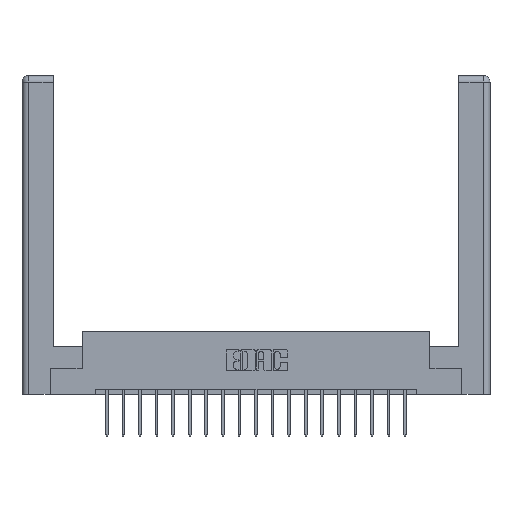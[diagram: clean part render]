
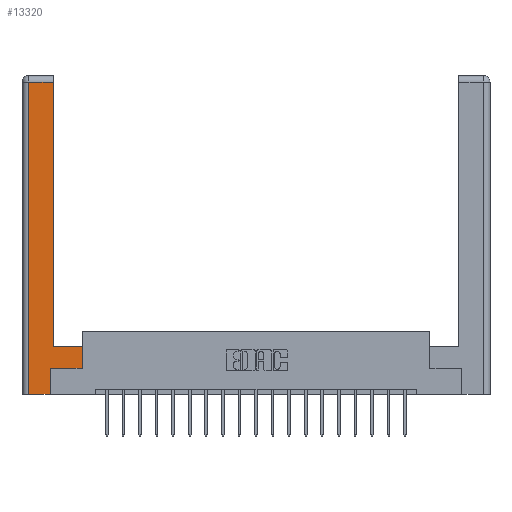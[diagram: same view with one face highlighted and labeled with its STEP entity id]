
A CAD part, top view. The second image highlights one B-rep face of the part: STEP entity #13320.
In plain terms, the highlighted planar face has unit normal (0, 0, 1).
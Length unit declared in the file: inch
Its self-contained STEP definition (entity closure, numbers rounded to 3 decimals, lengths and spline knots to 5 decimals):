
#683 = CARTESIAN_POINT ( 'NONE',  ( 0.295, 0.45, 0. ) ) ;
#913 = VECTOR ( 'NONE', #14217, 39.37008 ) ;
#1145 = CARTESIAN_POINT ( 'NONE',  ( 0.565, 0.245, 0. ) ) ;
#1337 = VERTEX_POINT ( 'NONE', #8075 ) ;
#1497 = DIRECTION ( 'NONE',  ( 0., -1., 0. ) ) ;
#1856 = CARTESIAN_POINT ( 'NONE',  ( 0.295, 2.94, 0. ) ) ;
#2027 = CARTESIAN_POINT ( 'NONE',  ( 0.565, 0.45, 0. ) ) ;
#2874 = EDGE_CURVE ( 'NONE', #4989, #14697, #19048, .T. ) ;
#3342 = ORIENTED_EDGE ( 'NONE', *, *, #14448, .T. ) ;
#3668 = DIRECTION ( 'NONE',  ( -1., 0., 0. ) ) ;
#3799 = PLANE ( 'NONE',  #14968 ) ;
#3950 = EDGE_CURVE ( 'NONE', #11197, #4989, #19739, .T. ) ;
#4392 = LINE ( 'NONE', #13558, #9795 ) ;
#4989 = VERTEX_POINT ( 'NONE', #2027 ) ;
#5073 = VECTOR ( 'NONE', #1497, 39.37008 ) ;
#5989 = EDGE_CURVE ( 'NONE', #13830, #11197, #15475, .T. ) ;
#6300 = ORIENTED_EDGE ( 'NONE', *, *, #15466, .T. ) ;
#6394 = VECTOR ( 'NONE', #11807, 39.37008 ) ;
#7390 = VERTEX_POINT ( 'NONE', #1856 ) ;
#7512 = EDGE_CURVE ( 'NONE', #1337, #7994, #4392, .T. ) ;
#7767 = CARTESIAN_POINT ( 'NONE',  ( 0.565, 0.45, 0. ) ) ;
#7864 = CARTESIAN_POINT ( 'NONE',  ( 0.0615, 2.94, 0. ) ) ;
#7979 = VECTOR ( 'NONE', #8437, 39.37008 ) ;
#7994 = VERTEX_POINT ( 'NONE', #13193 ) ;
#8042 = CARTESIAN_POINT ( 'NONE',  ( 0.265, 0.245, 0. ) ) ;
#8075 = CARTESIAN_POINT ( 'NONE',  ( 0.0615, 0., 0. ) ) ;
#8390 = CARTESIAN_POINT ( 'NONE',  ( 0., 0., 0. ) ) ;
#8437 = DIRECTION ( 'NONE',  ( 0., 1., 0. ) ) ;
#9795 = VECTOR ( 'NONE', #15606, 39.37008 ) ;
#9965 = LINE ( 'NONE', #17847, #7979 ) ;
#10145 = CARTESIAN_POINT ( 'NONE',  ( 0.295, 0.45, 0. ) ) ;
#10151 = DIRECTION ( 'NONE',  ( -1., 0., 0. ) ) ;
#10234 = ORIENTED_EDGE ( 'NONE', *, *, #16646, .T. ) ;
#11197 = VERTEX_POINT ( 'NONE', #1145 ) ;
#11807 = DIRECTION ( 'NONE',  ( 1., 0., 0. ) ) ;
#12295 = LINE ( 'NONE', #17549, #913 ) ;
#12521 = DIRECTION ( 'NONE',  ( 0., 1., 0. ) ) ;
#12589 = ORIENTED_EDGE ( 'NONE', *, *, #7512, .T. ) ;
#13193 = CARTESIAN_POINT ( 'NONE',  ( 0.265, 0., 0. ) ) ;
#13274 = ORIENTED_EDGE ( 'NONE', *, *, #2874, .T. ) ;
#13320 = ADVANCED_FACE ( 'NONE', ( #18961 ), #3799, .F. ) ;
#13558 = CARTESIAN_POINT ( 'NONE',  ( 0.265, 0., 0. ) ) ;
#13775 = EDGE_LOOP ( 'NONE', ( #19426, #3342, #10234, #12589, #6300, #20133, #18756, #13274 ) ) ;
#13830 = VERTEX_POINT ( 'NONE', #8042 ) ;
#14083 = CARTESIAN_POINT ( 'NONE',  ( 0.265, 0.245, 0. ) ) ;
#14217 = DIRECTION ( 'NONE',  ( -1., 0., 0. ) ) ;
#14448 = EDGE_CURVE ( 'NONE', #7390, #19556, #12295, .T. ) ;
#14459 = VECTOR ( 'NONE', #18677, 39.37008 ) ;
#14697 = VERTEX_POINT ( 'NONE', #10145 ) ;
#14786 = DIRECTION ( 'NONE',  ( 0., 0., -1. ) ) ;
#14968 = AXIS2_PLACEMENT_3D ( 'NONE', #8390, #14786, #3668 ) ;
#15466 = EDGE_CURVE ( 'NONE', #7994, #13830, #17133, .T. ) ;
#15475 = LINE ( 'NONE', #19473, #6394 ) ;
#15476 = CARTESIAN_POINT ( 'NONE',  ( 0.0615, 0., 0. ) ) ;
#15606 = DIRECTION ( 'NONE',  ( 1., 0., 0. ) ) ;
#16063 = VECTOR ( 'NONE', #12521, 39.37008 ) ;
#16646 = EDGE_CURVE ( 'NONE', #19556, #1337, #20274, .T. ) ;
#17133 = LINE ( 'NONE', #14083, #14459 ) ;
#17549 = CARTESIAN_POINT ( 'NONE',  ( 0.0615, 2.94, 0. ) ) ;
#17847 = CARTESIAN_POINT ( 'NONE',  ( 0.295, 3., 0. ) ) ;
#18294 = VECTOR ( 'NONE', #10151, 39.37008 ) ;
#18677 = DIRECTION ( 'NONE',  ( 0., 1., 0. ) ) ;
#18756 = ORIENTED_EDGE ( 'NONE', *, *, #3950, .T. ) ;
#18961 = FACE_OUTER_BOUND ( 'NONE', #13775, .T. ) ;
#19048 = LINE ( 'NONE', #683, #18294 ) ;
#19426 = ORIENTED_EDGE ( 'NONE', *, *, #20299, .T. ) ;
#19473 = CARTESIAN_POINT ( 'NONE',  ( 0.565, 0.245, 0. ) ) ;
#19556 = VERTEX_POINT ( 'NONE', #7864 ) ;
#19739 = LINE ( 'NONE', #7767, #16063 ) ;
#20133 = ORIENTED_EDGE ( 'NONE', *, *, #5989, .T. ) ;
#20274 = LINE ( 'NONE', #15476, #5073 ) ;
#20299 = EDGE_CURVE ( 'NONE', #14697, #7390, #9965, .T. ) ;
